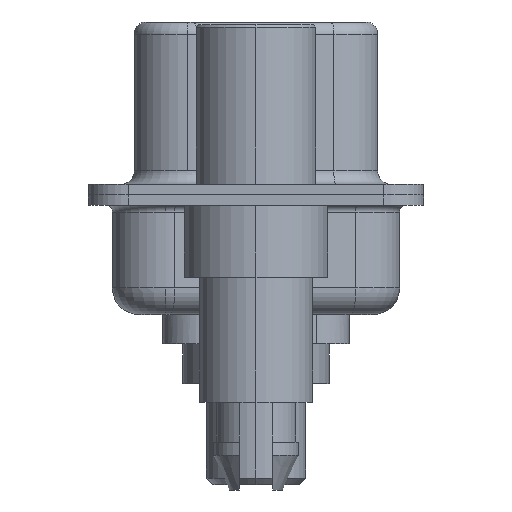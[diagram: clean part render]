
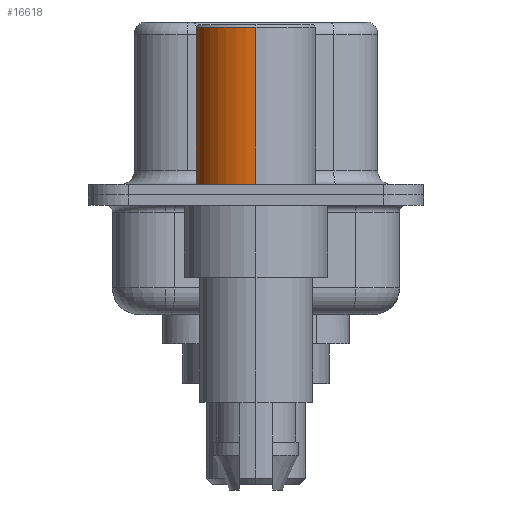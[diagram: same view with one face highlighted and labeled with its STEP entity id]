
A CAD part, left-side view. The second image highlights one B-rep face of the part: STEP entity #16618.
In plain terms, the highlighted cylindrical face has radius 2.25 mm (diameter 4.5 mm), a partial arc.
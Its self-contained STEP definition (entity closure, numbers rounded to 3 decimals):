
#907 = AXIS2_PLACEMENT_3D ( 'NONE', #979, #10657, #2352 ) ;
#973 = CARTESIAN_POINT ( 'NONE',  ( 2.25, 0., 6.3 ) ) ;
#979 = CARTESIAN_POINT ( 'NONE',  ( 0., 0., 0.4 ) ) ;
#1011 = DIRECTION ( 'NONE',  ( 1., 0., 0. ) ) ;
#1510 = VECTOR ( 'NONE', #3995, 1000. ) ;
#1650 = EDGE_CURVE ( 'NONE', #12455, #15734, #8820, .T. ) ;
#2352 = DIRECTION ( 'NONE',  ( 1., 0., 0. ) ) ;
#3995 = DIRECTION ( 'NONE',  ( 0., 0., 1. ) ) ;
#4158 = FACE_OUTER_BOUND ( 'NONE', #16341, .T. ) ;
#4286 = AXIS2_PLACEMENT_3D ( 'NONE', #10882, #5259, #12289 ) ;
#5259 = DIRECTION ( 'NONE',  ( 0., 0., 1. ) ) ;
#5501 = EDGE_CURVE ( 'NONE', #10363, #17460, #9580, .T. ) ;
#5709 = EDGE_CURVE ( 'NONE', #10363, #12455, #17191, .T. ) ;
#6495 = CYLINDRICAL_SURFACE ( 'NONE', #4286, 2.25 ) ;
#8820 = LINE ( 'NONE', #11105, #1510 ) ;
#9187 = ORIENTED_EDGE ( 'NONE', *, *, #13053, .F. ) ;
#9253 = DIRECTION ( 'NONE',  ( 0., 0., 1. ) ) ;
#9580 = LINE ( 'NONE', #11034, #10479 ) ;
#9586 = DIRECTION ( 'NONE',  ( 0., 0., 1. ) ) ;
#10294 = CARTESIAN_POINT ( 'NONE',  ( -2.25, 0., 0.4 ) ) ;
#10363 = VERTEX_POINT ( 'NONE', #11875 ) ;
#10479 = VECTOR ( 'NONE', #9586, 1000. ) ;
#10657 = DIRECTION ( 'NONE',  ( 0., 0., 1. ) ) ;
#10882 = CARTESIAN_POINT ( 'NONE',  ( 0., 0., 0.581 ) ) ;
#11034 = CARTESIAN_POINT ( 'NONE',  ( 2.25, 0., 0.581 ) ) ;
#11105 = CARTESIAN_POINT ( 'NONE',  ( -2.25, 0., 0.581 ) ) ;
#11875 = CARTESIAN_POINT ( 'NONE',  ( 2.25, 0., 0.4 ) ) ;
#12289 = DIRECTION ( 'NONE',  ( 1., 0., 0. ) ) ;
#12455 = VERTEX_POINT ( 'NONE', #10294 ) ;
#13053 = EDGE_CURVE ( 'NONE', #17460, #15734, #15993, .T. ) ;
#15734 = VERTEX_POINT ( 'NONE', #17301 ) ;
#15993 = CIRCLE ( 'NONE', #17250, 2.25 ) ;
#16072 = ORIENTED_EDGE ( 'NONE', *, *, #5501, .F. ) ;
#16259 = ORIENTED_EDGE ( 'NONE', *, *, #5709, .T. ) ;
#16341 = EDGE_LOOP ( 'NONE', ( #16259, #17503, #9187, #16072 ) ) ;
#16618 = ADVANCED_FACE ( 'NONE', ( #4158 ), #6495, .T. ) ;
#17191 = CIRCLE ( 'NONE', #907, 2.25 ) ;
#17250 = AXIS2_PLACEMENT_3D ( 'NONE', #17591, #9253, #1011 ) ;
#17301 = CARTESIAN_POINT ( 'NONE',  ( -2.25, 0., 6.3 ) ) ;
#17460 = VERTEX_POINT ( 'NONE', #973 ) ;
#17503 = ORIENTED_EDGE ( 'NONE', *, *, #1650, .T. ) ;
#17591 = CARTESIAN_POINT ( 'NONE',  ( 0., 0., 6.3 ) ) ;
